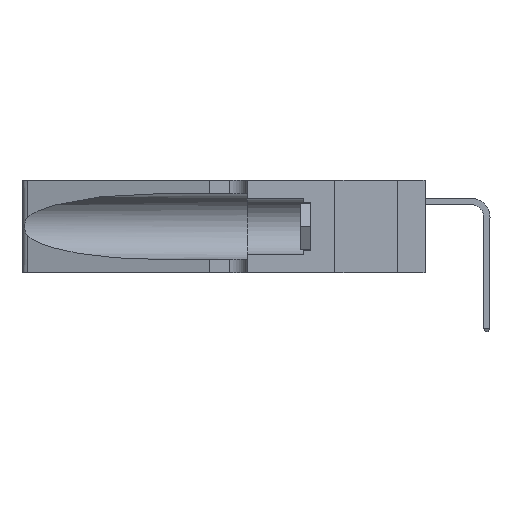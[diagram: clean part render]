
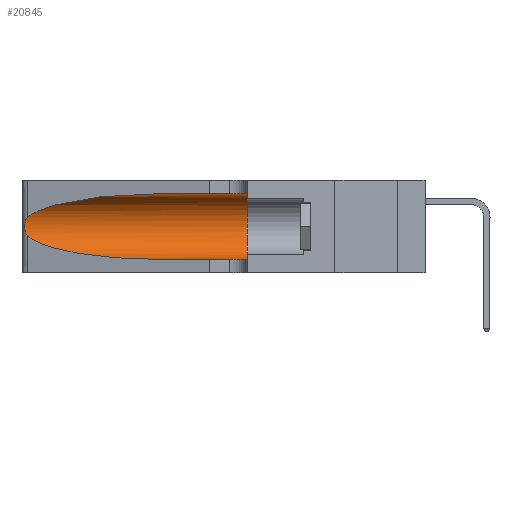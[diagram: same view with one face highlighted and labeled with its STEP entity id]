
A CAD part, left-side view. The second image highlights one B-rep face of the part: STEP entity #20845.
In plain terms, the highlighted cylindrical face has radius 3.308 mm (diameter 6.617 mm), a partial arc.
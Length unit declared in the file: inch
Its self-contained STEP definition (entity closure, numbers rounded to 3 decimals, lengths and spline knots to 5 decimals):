
#13 = CARTESIAN_POINT ( 'NONE',  ( 0.25487, 1.22718, 0.14631 ) ) ;
#369 =( BOUNDED_CURVE ( )  B_SPLINE_CURVE ( 3, ( #1763, #17160, #3570, #15525 ),
 .UNSPECIFIED., .F., .F. ) 
 B_SPLINE_CURVE_WITH_KNOTS ( ( 4, 4 ),
 ( 3.44316, 4.71239 ),
 .UNSPECIFIED. ) 
 CURVE ( )  GEOMETRIC_REPRESENTATION_ITEM ( )  RATIONAL_B_SPLINE_CURVE ( ( 1., 0.87, 0.87, 1. ) ) 
 REPRESENTATION_ITEM ( '' )  );
#385 = ORIENTED_EDGE ( 'NONE', *, *, #6757, .T. ) ;
#1031 = CARTESIAN_POINT ( 'NONE',  ( 0.2373, 1.15595, 0.28018 ) ) ;
#1215 = EDGE_CURVE ( 'NONE', #8600, #16325, #11872, .T. ) ;
#1518 = DIRECTION ( 'NONE',  ( 0., -1., 0. ) ) ;
#1760 = CARTESIAN_POINT ( 'NONE',  ( 0.1305, 0.35, 0.185 ) ) ;
#1763 = CARTESIAN_POINT ( 'NONE',  ( 0.25487, 1.22718, 0.14631 ) ) ;
#1784 = CARTESIAN_POINT ( 'NONE',  ( 0.25639, 1.23184, 0.21858 ) ) ;
#2374 = VERTEX_POINT ( 'NONE', #18275 ) ;
#2857 = DIRECTION ( 'NONE',  ( 0., -1., 0. ) ) ;
#3334 = CYLINDRICAL_SURFACE ( 'NONE', #15996, 0.13025 ) ;
#3570 = CARTESIAN_POINT ( 'NONE',  ( 0.18966, 0.96281, 0.05475 ) ) ;
#3591 = CARTESIAN_POINT ( 'NONE',  ( 0.25854, 1.2359, 0.20912 ) ) ;
#4196 = ORIENTED_EDGE ( 'NONE', *, *, #5092, .F. ) ;
#5044 = LINE ( 'NONE', #16931, #18027 ) ;
#5092 = EDGE_CURVE ( 'NONE', #22050, #8600, #5044, .T. ) ;
#5411 = CARTESIAN_POINT ( 'NONE',  ( 0.26075, 1.23896, 0.19203 ) ) ;
#5564 = DIRECTION ( 'NONE',  ( 0., -1., 0. ) ) ;
#6757 = EDGE_CURVE ( 'NONE', #2374, #6982, #369, .T. ) ;
#6982 = VERTEX_POINT ( 'NONE', #17806 ) ;
#7121 = CARTESIAN_POINT ( 'NONE',  ( 0.26017, 1.23833, 0.17102 ) ) ;
#7646 = EDGE_LOOP ( 'NONE', ( #13098, #14127, #385, #9789, #20875, #4196 ) ) ;
#8547 = FACE_OUTER_BOUND ( 'NONE', #7646, .T. ) ;
#8600 = VERTEX_POINT ( 'NONE', #21606 ) ;
#8781 = CARTESIAN_POINT ( 'NONE',  ( 0.25555, 1.22994, 0.2215 ) ) ;
#8850 = CARTESIAN_POINT ( 'NONE',  ( 0.25789, 1.23486, 0.15765 ) ) ;
#8990 = VERTEX_POINT ( 'NONE', #21001 ) ;
#9520 = EDGE_CURVE ( 'NONE', #6982, #16325, #19073, .T. ) ;
#9781 = CARTESIAN_POINT ( 'NONE',  ( 0.1305, 0.72297, 0.31525 ) ) ;
#9789 = ORIENTED_EDGE ( 'NONE', *, *, #9520, .T. ) ;
#10009 = B_SPLINE_CURVE_WITH_KNOTS ( 'NONE', 3,
 ( #22240, #8781, #1784, #13869, #3591, #15546, #5411, #17250, #7121, #18934, #8850, #20619, #10555, #13 ),
 .UNSPECIFIED., .F., .F.,
 ( 4, 2, 2, 2, 2, 2, 4 ),
 ( 0., 0.00027, 0.00053, 0.00107, 0.0016, 0.00187, 0.00214 ),
 .UNSPECIFIED. ) ;
#10555 = CARTESIAN_POINT ( 'NONE',  ( 0.25555, 1.22993, 0.14849 ) ) ;
#11492 = CARTESIAN_POINT ( 'NONE',  ( 0.1305, 1.61858, 0.185 ) ) ;
#11872 = CIRCLE ( 'NONE', #15237, 0.13025 ) ;
#13098 = ORIENTED_EDGE ( 'NONE', *, *, #17061, .T. ) ;
#13162 = CARTESIAN_POINT ( 'NONE',  ( 0.25487, 1.22718, 0.22369 ) ) ;
#13587 = EDGE_CURVE ( 'NONE', #8990, #2374, #10009, .T. ) ;
#13869 = CARTESIAN_POINT ( 'NONE',  ( 0.25787, 1.23484, 0.2124 ) ) ;
#14011 = CARTESIAN_POINT ( 'NONE',  ( 0.1305, 1.61858, 0.05475 ) ) ;
#14127 = ORIENTED_EDGE ( 'NONE', *, *, #13587, .T. ) ;
#15065 = CARTESIAN_POINT ( 'NONE',  ( 0.1305, 0.72297, 0.31525 ) ) ;
#15237 = AXIS2_PLACEMENT_3D ( 'NONE', #1760, #17158, #16779 ) ;
#15525 = CARTESIAN_POINT ( 'NONE',  ( 0.1305, 0.72297, 0.05475 ) ) ;
#15546 = CARTESIAN_POINT ( 'NONE',  ( 0.26018, 1.23835, 0.19895 ) ) ;
#15996 = AXIS2_PLACEMENT_3D ( 'NONE', #11492, #2857, #16566 ) ;
#16266 = CARTESIAN_POINT ( 'NONE',  ( 0.1305, 0.35, 0.05475 ) ) ;
#16325 = VERTEX_POINT ( 'NONE', #16266 ) ;
#16566 = DIRECTION ( 'NONE',  ( 0., 0., -1. ) ) ;
#16779 = DIRECTION ( 'NONE',  ( 0., 0., 1. ) ) ;
#16931 = CARTESIAN_POINT ( 'NONE',  ( 0.1305, 1.61858, 0.31525 ) ) ;
#17061 = EDGE_CURVE ( 'NONE', #22050, #8990, #20128, .T. ) ;
#17158 = DIRECTION ( 'NONE',  ( 0., 1., 0. ) ) ;
#17160 = CARTESIAN_POINT ( 'NONE',  ( 0.2373, 1.15595, 0.08982 ) ) ;
#17250 = CARTESIAN_POINT ( 'NONE',  ( 0.26075, 1.23896, 0.178 ) ) ;
#17806 = CARTESIAN_POINT ( 'NONE',  ( 0.1305, 0.72297, 0.05475 ) ) ;
#18027 = VECTOR ( 'NONE', #1518, 39.37008 ) ;
#18275 = CARTESIAN_POINT ( 'NONE',  ( 0.25487, 1.22718, 0.14631 ) ) ;
#18934 = CARTESIAN_POINT ( 'NONE',  ( 0.25856, 1.23593, 0.16098 ) ) ;
#19073 = LINE ( 'NONE', #14011, #21961 ) ;
#19856 = CARTESIAN_POINT ( 'NONE',  ( 0.18966, 0.96281, 0.31525 ) ) ;
#20128 =( BOUNDED_CURVE ( )  B_SPLINE_CURVE ( 3, ( #9781, #19856, #1031, #13162 ),
 .UNSPECIFIED., .F., .F. ) 
 B_SPLINE_CURVE_WITH_KNOTS ( ( 4, 4 ),
 ( 1.5708, 2.84003 ),
 .UNSPECIFIED. ) 
 CURVE ( )  GEOMETRIC_REPRESENTATION_ITEM ( )  RATIONAL_B_SPLINE_CURVE ( ( 1., 0.87, 0.87, 1. ) ) 
 REPRESENTATION_ITEM ( '' )  );
#20619 = CARTESIAN_POINT ( 'NONE',  ( 0.25639, 1.23186, 0.15144 ) ) ;
#20845 = ADVANCED_FACE ( 'NONE', ( #8547 ), #3334, .F. ) ;
#20875 = ORIENTED_EDGE ( 'NONE', *, *, #1215, .F. ) ;
#21001 = CARTESIAN_POINT ( 'NONE',  ( 0.25487, 1.22718, 0.22369 ) ) ;
#21606 = CARTESIAN_POINT ( 'NONE',  ( 0.1305, 0.35, 0.31525 ) ) ;
#21961 = VECTOR ( 'NONE', #5564, 39.37008 ) ;
#22050 = VERTEX_POINT ( 'NONE', #15065 ) ;
#22240 = CARTESIAN_POINT ( 'NONE',  ( 0.25487, 1.22718, 0.22369 ) ) ;
